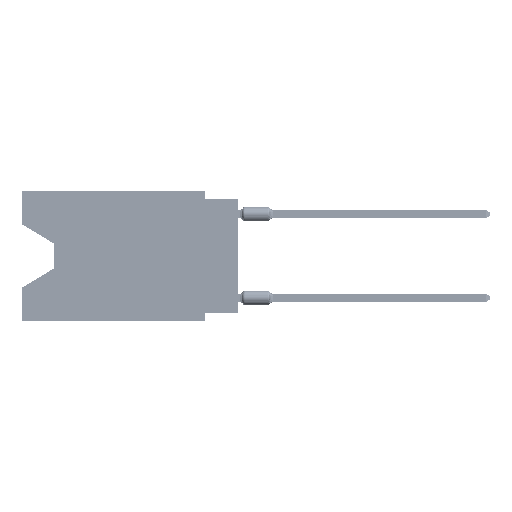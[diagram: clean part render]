
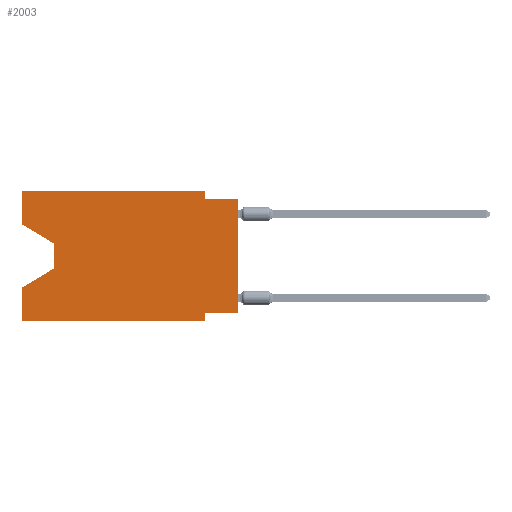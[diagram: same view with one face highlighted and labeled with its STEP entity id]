
A CAD part, left-side view. The second image highlights one B-rep face of the part: STEP entity #2003.
In plain terms, the highlighted planar face has unit normal (-1, 0, 0).
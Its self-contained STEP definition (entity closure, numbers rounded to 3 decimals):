
#2003 = ADVANCED_FACE ( 'NONE', ( #9450 ), #2295, .F. ) ;
#2159 = LINE ( 'NONE', #74753, #8849 ) ;
#2295 = PLANE ( 'NONE',  #5417 ) ;
#3461 = EDGE_CURVE ( 'NONE', #63240, #46475, #14352, .T. ) ;
#5417 = AXIS2_PLACEMENT_3D ( 'NONE', #63329, #45382, #15056 ) ;
#5864 = ORIENTED_EDGE ( 'NONE', *, *, #30087, .F. ) ;
#6517 = CARTESIAN_POINT ( 'NONE',  ( 0., 13.97, -4.013 ) ) ;
#7065 = ORIENTED_EDGE ( 'NONE', *, *, #32721, .T. ) ;
#8849 = VECTOR ( 'NONE', #31722, 1000. ) ;
#9091 = ORIENTED_EDGE ( 'NONE', *, *, #11541, .F. ) ;
#9450 = FACE_OUTER_BOUND ( 'NONE', #59810, .T. ) ;
#10043 = CARTESIAN_POINT ( 'NONE',  ( 0., 0., 0. ) ) ;
#11150 = EDGE_CURVE ( 'NONE', #15393, #60284, #18499, .T. ) ;
#11254 = ORIENTED_EDGE ( 'NONE', *, *, #76300, .T. ) ;
#11541 = EDGE_CURVE ( 'NONE', #13920, #63240, #33341, .T. ) ;
#12526 = DIRECTION ( 'NONE',  ( 0., 0., -1. ) ) ;
#12981 = VERTEX_POINT ( 'NONE', #77618 ) ;
#13077 = CARTESIAN_POINT ( 'NONE',  ( 0., 16.383, 0. ) ) ;
#13920 = VERTEX_POINT ( 'NONE', #51523 ) ;
#14352 = LINE ( 'NONE', #57815, #66700 ) ;
#15056 = DIRECTION ( 'NONE',  ( 0., 0., -1. ) ) ;
#15390 = VECTOR ( 'NONE', #76263, 1000. ) ;
#15393 = VERTEX_POINT ( 'NONE', #73235 ) ;
#15548 = LINE ( 'NONE', #75788, #41614 ) ;
#15746 = CARTESIAN_POINT ( 'NONE',  ( 0., 0., -0.635 ) ) ;
#16102 = CARTESIAN_POINT ( 'NONE',  ( 0., 13.97, -5.893 ) ) ;
#17025 = VECTOR ( 'NONE', #25636, 1000. ) ;
#17189 = DIRECTION ( 'NONE',  ( 0., -0.855, -0.519 ) ) ;
#18499 = LINE ( 'NONE', #38025, #77634 ) ;
#19904 = ORIENTED_EDGE ( 'NONE', *, *, #26055, .T. ) ;
#21278 = VERTEX_POINT ( 'NONE', #64972 ) ;
#22289 = CARTESIAN_POINT ( 'NONE',  ( 0., 0., -0.635 ) ) ;
#22944 = ORIENTED_EDGE ( 'NONE', *, *, #47531, .T. ) ;
#25636 = DIRECTION ( 'NONE',  ( 0., -1., 0. ) ) ;
#25798 = EDGE_CURVE ( 'NONE', #37708, #15393, #62686, .T. ) ;
#25915 = VECTOR ( 'NONE', #61177, 1000. ) ;
#26055 = EDGE_CURVE ( 'NONE', #12981, #21278, #66233, .T. ) ;
#26984 = ORIENTED_EDGE ( 'NONE', *, *, #11150, .F. ) ;
#28198 = VECTOR ( 'NONE', #41419, 1000. ) ;
#29222 = ORIENTED_EDGE ( 'NONE', *, *, #63204, .T. ) ;
#30087 = EDGE_CURVE ( 'NONE', #60284, #51303, #76926, .T. ) ;
#31570 = CARTESIAN_POINT ( 'NONE',  ( 0., 16.383, 0. ) ) ;
#31722 = DIRECTION ( 'NONE',  ( 0., 0.855, -0.519 ) ) ;
#32721 = EDGE_CURVE ( 'NONE', #21278, #58339, #78347, .T. ) ;
#33341 = LINE ( 'NONE', #44920, #73858 ) ;
#35546 = CARTESIAN_POINT ( 'NONE',  ( 0., 16.383, -2.546 ) ) ;
#36539 = ORIENTED_EDGE ( 'NONE', *, *, #25798, .F. ) ;
#36658 = EDGE_CURVE ( 'NONE', #60403, #53168, #48995, .T. ) ;
#37708 = VERTEX_POINT ( 'NONE', #31570 ) ;
#38025 = CARTESIAN_POINT ( 'NONE',  ( 0., 2.54, 0. ) ) ;
#38696 = CARTESIAN_POINT ( 'NONE',  ( 0., 16.383, -9.906 ) ) ;
#38698 = VECTOR ( 'NONE', #78244, 1000. ) ;
#39048 = ORIENTED_EDGE ( 'NONE', *, *, #3461, .F. ) ;
#40775 = EDGE_CURVE ( 'NONE', #12981, #37708, #15548, .T. ) ;
#40777 = LINE ( 'NONE', #53915, #38698 ) ;
#41419 = DIRECTION ( 'NONE',  ( 0., -1., 0. ) ) ;
#41614 = VECTOR ( 'NONE', #56264, 1000. ) ;
#44920 = CARTESIAN_POINT ( 'NONE',  ( 0., 0., -9.271 ) ) ;
#45382 = DIRECTION ( 'NONE',  ( 1., 0., 0. ) ) ;
#46475 = VERTEX_POINT ( 'NONE', #57100 ) ;
#47076 = CARTESIAN_POINT ( 'NONE',  ( 0., 16.383, -7.36 ) ) ;
#47531 = EDGE_CURVE ( 'NONE', #13920, #51303, #51133, .T. ) ;
#48995 = LINE ( 'NONE', #13077, #56692 ) ;
#49181 = CARTESIAN_POINT ( 'NONE',  ( 0., 16.383, 0. ) ) ;
#51055 = DIRECTION ( 'NONE',  ( 0., 0., -1. ) ) ;
#51133 = LINE ( 'NONE', #10043, #15390 ) ;
#51303 = VERTEX_POINT ( 'NONE', #15746 ) ;
#51523 = CARTESIAN_POINT ( 'NONE',  ( 0., 0., -9.271 ) ) ;
#51880 = ORIENTED_EDGE ( 'NONE', *, *, #40775, .F. ) ;
#53168 = VERTEX_POINT ( 'NONE', #47076 ) ;
#53915 = CARTESIAN_POINT ( 'NONE',  ( 0., 16.383, -9.906 ) ) ;
#54353 = ORIENTED_EDGE ( 'NONE', *, *, #36658, .F. ) ;
#55766 = DIRECTION ( 'NONE',  ( 0., 0., 1. ) ) ;
#56111 = DIRECTION ( 'NONE',  ( 0., 1., 0. ) ) ;
#56264 = DIRECTION ( 'NONE',  ( 0., 0., 1. ) ) ;
#56692 = VECTOR ( 'NONE', #55766, 1000. ) ;
#57100 = CARTESIAN_POINT ( 'NONE',  ( 0., 2.54, -9.906 ) ) ;
#57815 = CARTESIAN_POINT ( 'NONE',  ( 0., 2.54, -9.906 ) ) ;
#58339 = VERTEX_POINT ( 'NONE', #16102 ) ;
#59810 = EDGE_LOOP ( 'NONE', ( #19904, #7065, #29222, #54353, #11254, #39048, #9091, #22944, #5864, #26984, #36539, #51880 ) ) ;
#60284 = VERTEX_POINT ( 'NONE', #68196 ) ;
#60403 = VERTEX_POINT ( 'NONE', #38696 ) ;
#61177 = DIRECTION ( 'NONE',  ( 0., 0., -1. ) ) ;
#62686 = LINE ( 'NONE', #49181, #17025 ) ;
#63204 = EDGE_CURVE ( 'NONE', #58339, #53168, #2159, .T. ) ;
#63240 = VERTEX_POINT ( 'NONE', #73977 ) ;
#63329 = CARTESIAN_POINT ( 'NONE',  ( 0., 16.383, 0. ) ) ;
#64972 = CARTESIAN_POINT ( 'NONE',  ( 0., 13.97, -4.013 ) ) ;
#65473 = VECTOR ( 'NONE', #17189, 1000. ) ;
#66233 = LINE ( 'NONE', #35546, #65473 ) ;
#66700 = VECTOR ( 'NONE', #51055, 1000. ) ;
#68196 = CARTESIAN_POINT ( 'NONE',  ( 0., 2.54, -0.635 ) ) ;
#73235 = CARTESIAN_POINT ( 'NONE',  ( 0., 2.54, 0. ) ) ;
#73858 = VECTOR ( 'NONE', #56111, 1000. ) ;
#73977 = CARTESIAN_POINT ( 'NONE',  ( 0., 2.54, -9.271 ) ) ;
#74753 = CARTESIAN_POINT ( 'NONE',  ( 0., 13.97, -5.893 ) ) ;
#75788 = CARTESIAN_POINT ( 'NONE',  ( 0., 16.383, 0. ) ) ;
#76263 = DIRECTION ( 'NONE',  ( 0., 0., 1. ) ) ;
#76300 = EDGE_CURVE ( 'NONE', #60403, #46475, #40777, .T. ) ;
#76926 = LINE ( 'NONE', #22289, #28198 ) ;
#77618 = CARTESIAN_POINT ( 'NONE',  ( 0., 16.383, -2.546 ) ) ;
#77634 = VECTOR ( 'NONE', #12526, 1000. ) ;
#78244 = DIRECTION ( 'NONE',  ( 0., -1., 0. ) ) ;
#78347 = LINE ( 'NONE', #6517, #25915 ) ;
